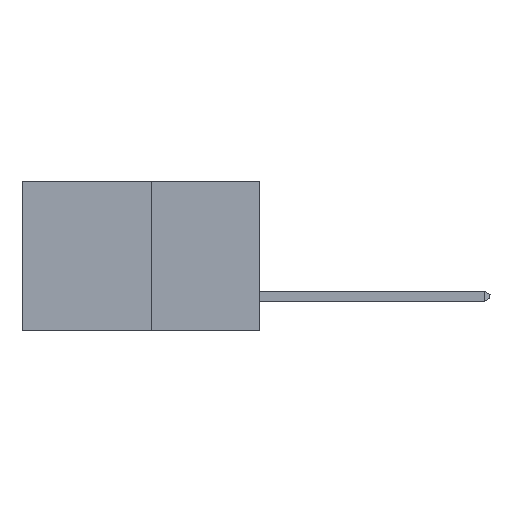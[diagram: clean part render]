
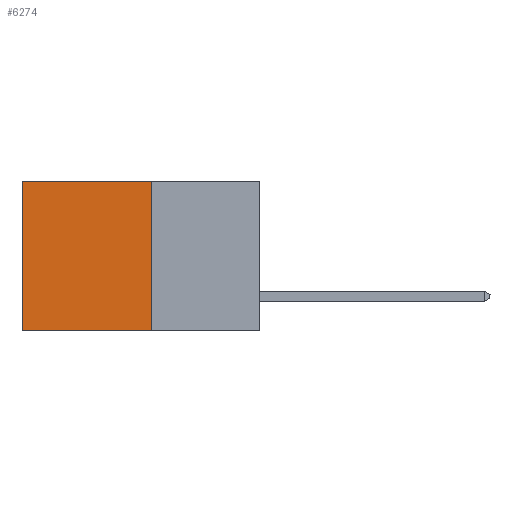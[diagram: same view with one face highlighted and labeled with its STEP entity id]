
A CAD part, left-side view. The second image highlights one B-rep face of the part: STEP entity #6274.
In plain terms, the highlighted planar face has unit normal (-1, 0, 0).
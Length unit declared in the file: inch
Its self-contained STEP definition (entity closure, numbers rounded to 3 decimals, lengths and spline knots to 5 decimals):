
#608 = DIRECTION ( 'NONE',  ( 0., 1., 0. ) ) ;
#965 = EDGE_CURVE ( 'NONE', #7296, #11246, #11241, .T. ) ;
#1036 = LINE ( 'NONE', #5285, #5802 ) ;
#1053 = VERTEX_POINT ( 'NONE', #11142 ) ;
#1482 = DIRECTION ( 'NONE',  ( 0., 1., 0. ) ) ;
#1573 = DIRECTION ( 'NONE',  ( 0., 0., -1. ) ) ;
#1702 = PLANE ( 'NONE',  #9212 ) ;
#1969 = VECTOR ( 'NONE', #1573, 39.37008 ) ;
#2601 = CARTESIAN_POINT ( 'NONE',  ( 0.277, 0.27, 0. ) ) ;
#2648 = CARTESIAN_POINT ( 'NONE',  ( 0.277, 0.27, -0.37 ) ) ;
#2787 = EDGE_CURVE ( 'NONE', #8183, #1053, #10628, .T. ) ;
#3232 = ORIENTED_EDGE ( 'NONE', *, *, #2787, .T. ) ;
#3407 = CARTESIAN_POINT ( 'NONE',  ( 0.277, 0.27, -0.37 ) ) ;
#3689 = DIRECTION ( 'NONE',  ( 0., 0., -1. ) ) ;
#4052 = EDGE_LOOP ( 'NONE', ( #3232, #5975, #10189, #8387 ) ) ;
#4263 = CARTESIAN_POINT ( 'NONE',  ( 0.277, 0.59, -0.37 ) ) ;
#4601 = DIRECTION ( 'NONE',  ( 0., 0., -1. ) ) ;
#5231 = LINE ( 'NONE', #2601, #5520 ) ;
#5285 = CARTESIAN_POINT ( 'NONE',  ( 0.277, 0.27, -0.37 ) ) ;
#5520 = VECTOR ( 'NONE', #608, 39.37008 ) ;
#5650 = CARTESIAN_POINT ( 'NONE',  ( 0.277, 0.27, 0. ) ) ;
#5802 = VECTOR ( 'NONE', #1482, 39.37008 ) ;
#5975 = ORIENTED_EDGE ( 'NONE', *, *, #8647, .F. ) ;
#6274 = ADVANCED_FACE ( 'NONE', ( #8616 ), #1702, .F. ) ;
#7296 = VERTEX_POINT ( 'NONE', #5650 ) ;
#8183 = VERTEX_POINT ( 'NONE', #10728 ) ;
#8387 = ORIENTED_EDGE ( 'NONE', *, *, #8954, .T. ) ;
#8572 = VECTOR ( 'NONE', #4601, 39.37008 ) ;
#8616 = FACE_OUTER_BOUND ( 'NONE', #4052, .T. ) ;
#8647 = EDGE_CURVE ( 'NONE', #11246, #1053, #1036, .T. ) ;
#8771 = DIRECTION ( 'NONE',  ( 1., 0., 0. ) ) ;
#8954 = EDGE_CURVE ( 'NONE', #7296, #8183, #5231, .T. ) ;
#9212 = AXIS2_PLACEMENT_3D ( 'NONE', #2648, #8771, #3689 ) ;
#10189 = ORIENTED_EDGE ( 'NONE', *, *, #965, .F. ) ;
#10628 = LINE ( 'NONE', #4263, #8572 ) ;
#10632 = CARTESIAN_POINT ( 'NONE',  ( 0.277, 0.27, -0.37 ) ) ;
#10728 = CARTESIAN_POINT ( 'NONE',  ( 0.277, 0.59, 0. ) ) ;
#11142 = CARTESIAN_POINT ( 'NONE',  ( 0.277, 0.59, -0.37 ) ) ;
#11241 = LINE ( 'NONE', #10632, #1969 ) ;
#11246 = VERTEX_POINT ( 'NONE', #3407 ) ;
